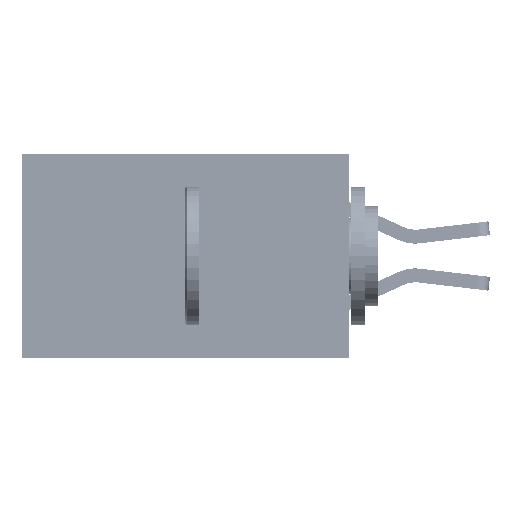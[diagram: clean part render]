
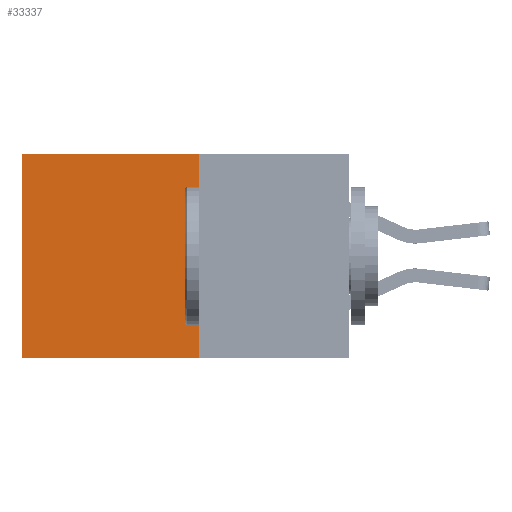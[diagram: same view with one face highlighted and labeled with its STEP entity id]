
A CAD part, left-side view. The second image highlights one B-rep face of the part: STEP entity #33337.
In plain terms, the highlighted planar face has unit normal (-1, 0, 0).
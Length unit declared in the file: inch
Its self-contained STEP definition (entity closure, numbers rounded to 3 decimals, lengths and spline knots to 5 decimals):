
#2010 = CARTESIAN_POINT ( 'NONE',  ( 0.277, 0.59, -0.37 ) ) ;
#3738 = ORIENTED_EDGE ( 'NONE', *, *, #27551, .T. ) ;
#4738 = CARTESIAN_POINT ( 'NONE',  ( 0.277, 0.59, 0. ) ) ;
#5376 = CARTESIAN_POINT ( 'NONE',  ( 0.277, 0.27, -0.37 ) ) ;
#5568 = PLANE ( 'NONE',  #21224 ) ;
#5683 = DIRECTION ( 'NONE',  ( 1., 0., 0. ) ) ;
#6361 = ORIENTED_EDGE ( 'NONE', *, *, #10487, .F. ) ;
#8692 = CARTESIAN_POINT ( 'NONE',  ( 0.277, 0.59, -0.37 ) ) ;
#10166 = CARTESIAN_POINT ( 'NONE',  ( 0.277, 0.27, -0.37 ) ) ;
#10391 = VERTEX_POINT ( 'NONE', #2010 ) ;
#10487 = EDGE_CURVE ( 'NONE', #22071, #15060, #19530, .T. ) ;
#10600 = CARTESIAN_POINT ( 'NONE',  ( 0.277, 0.27, -0.37 ) ) ;
#11331 = DIRECTION ( 'NONE',  ( 0., 0., -1. ) ) ;
#11693 = VECTOR ( 'NONE', #29028, 39.37008 ) ;
#12049 = ORIENTED_EDGE ( 'NONE', *, *, #27102, .F. ) ;
#12284 = DIRECTION ( 'NONE',  ( 0., 1., 0. ) ) ;
#12518 = LINE ( 'NONE', #10600, #11693 ) ;
#12779 = DIRECTION ( 'NONE',  ( 0., 0., -1. ) ) ;
#12788 = ORIENTED_EDGE ( 'NONE', *, *, #32177, .T. ) ;
#12911 = FACE_OUTER_BOUND ( 'NONE', #28005, .T. ) ;
#13320 = LINE ( 'NONE', #22817, #31877 ) ;
#15060 = VERTEX_POINT ( 'NONE', #5376 ) ;
#18695 = VECTOR ( 'NONE', #12779, 39.37008 ) ;
#18770 = VECTOR ( 'NONE', #11331, 39.37008 ) ;
#19530 = LINE ( 'NONE', #10166, #18695 ) ;
#21224 = AXIS2_PLACEMENT_3D ( 'NONE', #29248, #5683, #24098 ) ;
#22071 = VERTEX_POINT ( 'NONE', #27633 ) ;
#22817 = CARTESIAN_POINT ( 'NONE',  ( 0.277, 0.27, 0. ) ) ;
#24098 = DIRECTION ( 'NONE',  ( 0., 0., -1. ) ) ;
#24356 = VERTEX_POINT ( 'NONE', #4738 ) ;
#27102 = EDGE_CURVE ( 'NONE', #15060, #10391, #12518, .T. ) ;
#27551 = EDGE_CURVE ( 'NONE', #22071, #24356, #13320, .T. ) ;
#27633 = CARTESIAN_POINT ( 'NONE',  ( 0.277, 0.27, 0. ) ) ;
#28005 = EDGE_LOOP ( 'NONE', ( #12788, #12049, #6361, #3738 ) ) ;
#29028 = DIRECTION ( 'NONE',  ( 0., 1., 0. ) ) ;
#29248 = CARTESIAN_POINT ( 'NONE',  ( 0.277, 0.27, -0.37 ) ) ;
#31877 = VECTOR ( 'NONE', #12284, 39.37008 ) ;
#32177 = EDGE_CURVE ( 'NONE', #24356, #10391, #32807, .T. ) ;
#32807 = LINE ( 'NONE', #8692, #18770 ) ;
#33337 = ADVANCED_FACE ( 'NONE', ( #12911 ), #5568, .F. ) ;
